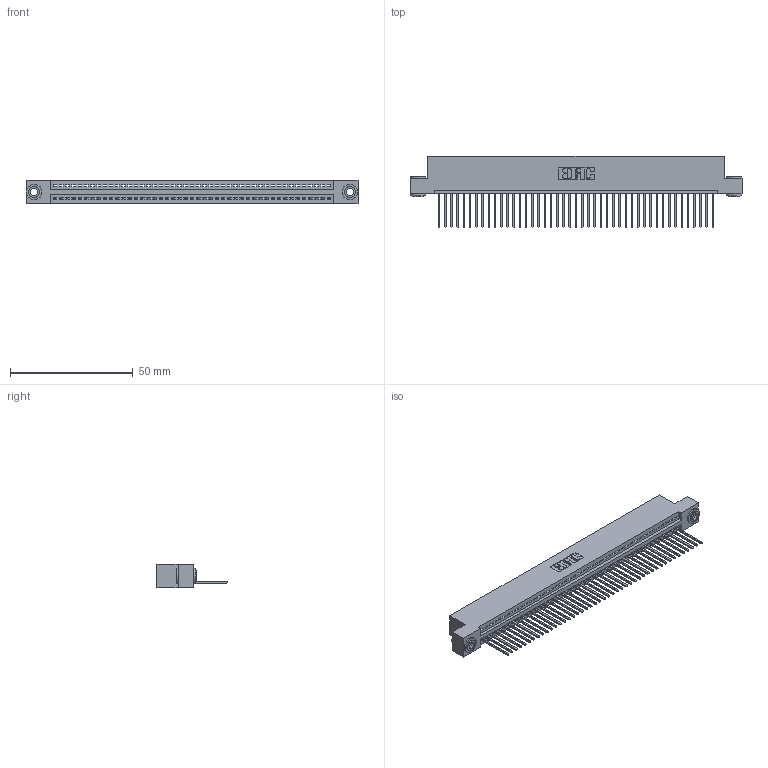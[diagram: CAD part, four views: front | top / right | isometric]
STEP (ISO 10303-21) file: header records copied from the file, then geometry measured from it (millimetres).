
FILE_DESCRIPTION (( 'STEP AP203' ), '1' );
FILE_NAME ('345-045-540-103.STEP', '2019-10-08T21:18:49', ( '' ), ( '' ), 'SwSTEP 2.0', 'SolidWorks 2016', '' );
FILE_SCHEMA (( 'CONFIG_CONTROL_DESIGN' ));
Length unit declared in the file: inch
Products named in the file (4): 345 Part_Flush Mounting Lugs - 0.156 Dia-TH; 345-250-002_345-250-002-102; 345-292-001_345-293-140; 345-045-540-103
Assembly tree (48 placements, depth 2):
  345-045-540-103
    345 Part_Flush Mounting Lugs - 0.156 Dia-TH
    345-292-001_345-293-140  x45
    345-250-002_345-250-002-102  x2
Bounding box: 135.51 x 29.13 x 9.4 mm (x, y, z)
Volume: 12975.7 mm3; surface area: 17937.2 mm2
Topology: 48 solids, 48 shells, 2774 faces, 8337 edges, 5494 vertices
Faces by surface type: plane 1890, cylinder 876, cone 8
Entity records: 34132 total; most frequent: CARTESIAN_POINT 5890, ORIENTED_EDGE 5862, DIRECTION 5171, EDGE_CURVE 2931, LINE 2595, VECTOR 2595, VERTEX_POINT 1950, AXIS2_PLACEMENT_3D 1288
